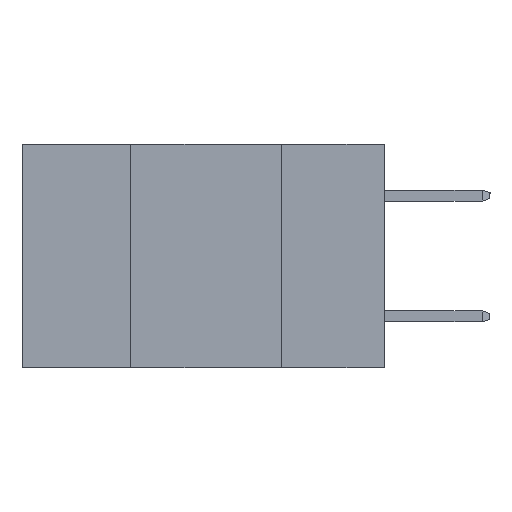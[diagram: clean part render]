
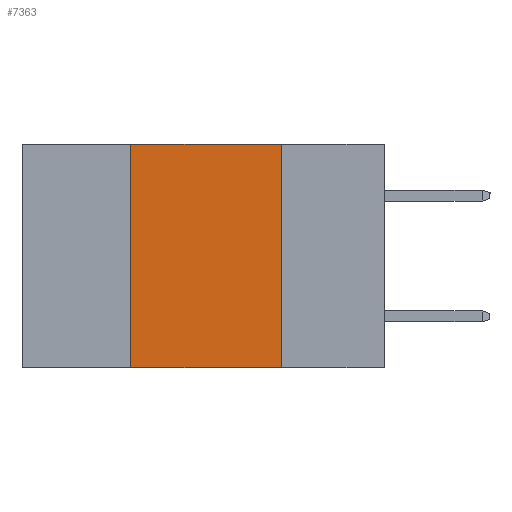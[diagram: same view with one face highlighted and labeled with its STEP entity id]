
A CAD part, left-side view. The second image highlights one B-rep face of the part: STEP entity #7363.
In plain terms, the highlighted planar face has unit normal (-1, 0, 0).
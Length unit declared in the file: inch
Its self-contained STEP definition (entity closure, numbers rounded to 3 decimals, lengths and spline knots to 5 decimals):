
#529 = LINE ( 'NONE', #2993, #8877 ) ;
#745 = FACE_OUTER_BOUND ( 'NONE', #1739, .T. ) ;
#1237 = ORIENTED_EDGE ( 'NONE', *, *, #3862, .F. ) ;
#1305 = ORIENTED_EDGE ( 'NONE', *, *, #2363, .F. ) ;
#1686 = CARTESIAN_POINT ( 'NONE',  ( 0., 0.6, 0. ) ) ;
#1739 = EDGE_LOOP ( 'NONE', ( #1237, #1305, #6722, #4542 ) ) ;
#1784 = DIRECTION ( 'NONE',  ( 0., -1., 0. ) ) ;
#1974 = VERTEX_POINT ( 'NONE', #2894 ) ;
#2310 = CARTESIAN_POINT ( 'NONE',  ( 0., 0.17, -0.37 ) ) ;
#2344 = VECTOR ( 'NONE', #3226, 39.37008 ) ;
#2361 = VERTEX_POINT ( 'NONE', #3994 ) ;
#2363 = EDGE_CURVE ( 'NONE', #2361, #4581, #3182, .T. ) ;
#2495 = CARTESIAN_POINT ( 'NONE',  ( 0., 0.6, 0. ) ) ;
#2789 = VECTOR ( 'NONE', #1784, 39.37008 ) ;
#2894 = CARTESIAN_POINT ( 'NONE',  ( 0., 0.42, -0.37 ) ) ;
#2917 = VERTEX_POINT ( 'NONE', #2310 ) ;
#2993 = CARTESIAN_POINT ( 'NONE',  ( 0., 0.6, -0.37 ) ) ;
#3182 = LINE ( 'NONE', #1686, #2789 ) ;
#3226 = DIRECTION ( 'NONE',  ( 0., 0., 1. ) ) ;
#3828 = DIRECTION ( 'NONE',  ( 1., 0., 0. ) ) ;
#3862 = EDGE_CURVE ( 'NONE', #4581, #2917, #9896, .T. ) ;
#3994 = CARTESIAN_POINT ( 'NONE',  ( 0., 0.42, 0. ) ) ;
#4511 = EDGE_CURVE ( 'NONE', #1974, #2917, #529, .T. ) ;
#4542 = ORIENTED_EDGE ( 'NONE', *, *, #4511, .T. ) ;
#4581 = VERTEX_POINT ( 'NONE', #7248 ) ;
#4739 = LINE ( 'NONE', #9650, #2344 ) ;
#6251 = EDGE_CURVE ( 'NONE', #1974, #2361, #4739, .T. ) ;
#6722 = ORIENTED_EDGE ( 'NONE', *, *, #6251, .F. ) ;
#7248 = CARTESIAN_POINT ( 'NONE',  ( 0., 0.17, 0. ) ) ;
#7363 = ADVANCED_FACE ( 'NONE', ( #745 ), #9638, .F. ) ;
#7838 = VECTOR ( 'NONE', #8588, 39.37008 ) ;
#8588 = DIRECTION ( 'NONE',  ( 0., 0., -1. ) ) ;
#8877 = VECTOR ( 'NONE', #10219, 39.37008 ) ;
#9123 = CARTESIAN_POINT ( 'NONE',  ( 0., 0.17, -0.37 ) ) ;
#9638 = PLANE ( 'NONE',  #9657 ) ;
#9650 = CARTESIAN_POINT ( 'NONE',  ( 0., 0.42, -0.37 ) ) ;
#9657 = AXIS2_PLACEMENT_3D ( 'NONE', #2495, #3828, #10234 ) ;
#9896 = LINE ( 'NONE', #9123, #7838 ) ;
#10219 = DIRECTION ( 'NONE',  ( 0., -1., 0. ) ) ;
#10234 = DIRECTION ( 'NONE',  ( 0., 0., -1. ) ) ;
